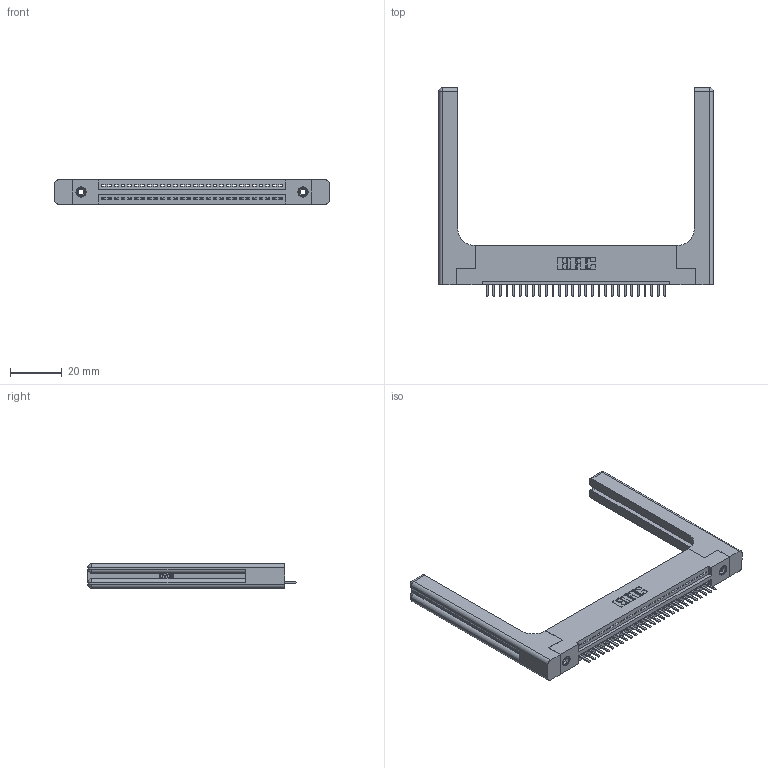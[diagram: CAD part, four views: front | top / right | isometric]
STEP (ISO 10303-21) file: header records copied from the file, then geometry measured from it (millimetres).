
FILE_DESCRIPTION (( 'STEP AP203' ), '1' );
FILE_NAME ('345-028-520-158.STEP', '2019-10-07T04:58:35', ( '' ), ( '' ), 'SwSTEP 2.0', 'SolidWorks 2016', '' );
FILE_SCHEMA (( 'CONFIG_CONTROL_DESIGN' ));
Length unit declared in the file: inch
Products named in the file (5): 345-028-520-158; 345-220-058_345-220-058; 345-250-001_345-250-001-102; 345 Part_Flush Mounting Lugs - 0.156 Dia-TH; 345-292-001_345-293-120
Assembly tree (33 placements, depth 2):
  345-028-520-158
    345 Part_Flush Mounting Lugs - 0.156 Dia-TH
    345-292-001_345-293-120  x28
    345-250-001_345-250-001-102  x2
    345-220-058_345-220-058  x2
Bounding box: 106.15 x 80.64 x 9.4 mm (x, y, z)
Volume: 18391.6 mm3; surface area: 17990.3 mm2
Topology: 33 solids, 33 shells, 2118 faces, 6159 edges, 4010 vertices
Faces by surface type: plane 1404, cylinder 654, bspline 36, cone 12, sphere 8, torus 4
Entity records: 28254 total; most frequent: CARTESIAN_POINT 5877, ORIENTED_EDGE 4624, DIRECTION 4088, EDGE_CURVE 2312, LINE 1972, VECTOR 1972, VERTEX_POINT 1530, AXIS2_PLACEMENT_3D 1058
